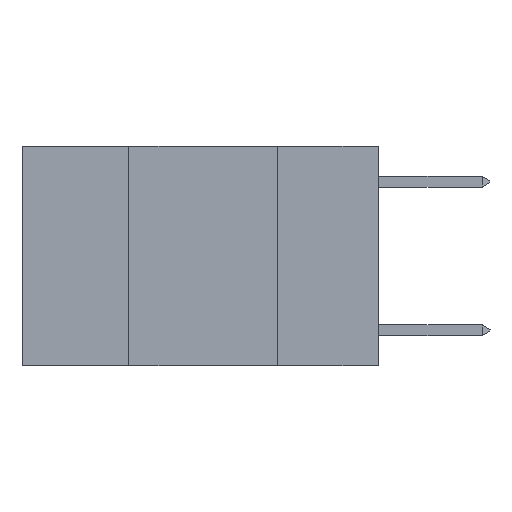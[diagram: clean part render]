
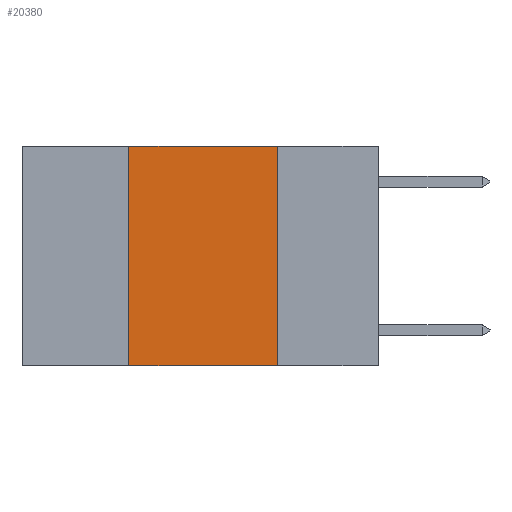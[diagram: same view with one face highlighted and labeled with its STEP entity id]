
A CAD part, left-side view. The second image highlights one B-rep face of the part: STEP entity #20380.
In plain terms, the highlighted planar face has unit normal (-1, 0, 0).
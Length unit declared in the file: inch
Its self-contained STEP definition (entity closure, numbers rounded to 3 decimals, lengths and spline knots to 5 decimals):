
#111 = DIRECTION ( 'NONE',  ( 1., 0., 0. ) ) ;
#132 = LINE ( 'NONE', #4312, #19120 ) ;
#354 = CARTESIAN_POINT ( 'NONE',  ( 0., 0.17, -0.37 ) ) ;
#672 = VERTEX_POINT ( 'NONE', #4099 ) ;
#1702 = CARTESIAN_POINT ( 'NONE',  ( 0., 0.17, 0. ) ) ;
#2691 = VECTOR ( 'NONE', #25414, 39.37008 ) ;
#3726 = DIRECTION ( 'NONE',  ( 0., 0., -1. ) ) ;
#4099 = CARTESIAN_POINT ( 'NONE',  ( 0., 0.42, 0. ) ) ;
#4312 = CARTESIAN_POINT ( 'NONE',  ( 0., 0.6, -0.37 ) ) ;
#4692 = DIRECTION ( 'NONE',  ( 0., 0., -1. ) ) ;
#7122 = LINE ( 'NONE', #19374, #2691 ) ;
#7652 = CARTESIAN_POINT ( 'NONE',  ( 0., 0.42, -0.37 ) ) ;
#8098 = ORIENTED_EDGE ( 'NONE', *, *, #11723, .T. ) ;
#8378 = DIRECTION ( 'NONE',  ( 0., -1., 0. ) ) ;
#8438 = VERTEX_POINT ( 'NONE', #354 ) ;
#8599 = EDGE_CURVE ( 'NONE', #26456, #672, #26024, .T. ) ;
#9667 = VECTOR ( 'NONE', #3726, 39.37008 ) ;
#9805 = EDGE_CURVE ( 'NONE', #672, #20671, #7122, .T. ) ;
#11723 = EDGE_CURVE ( 'NONE', #26456, #8438, #132, .T. ) ;
#13825 = DIRECTION ( 'NONE',  ( 0., 0., 1. ) ) ;
#13975 = LINE ( 'NONE', #22179, #9667 ) ;
#15125 = ORIENTED_EDGE ( 'NONE', *, *, #9805, .F. ) ;
#16006 = VECTOR ( 'NONE', #13825, 39.37008 ) ;
#17227 = AXIS2_PLACEMENT_3D ( 'NONE', #24736, #111, #4692 ) ;
#19120 = VECTOR ( 'NONE', #8378, 39.37008 ) ;
#19374 = CARTESIAN_POINT ( 'NONE',  ( 0., 0.6, 0. ) ) ;
#20332 = ORIENTED_EDGE ( 'NONE', *, *, #8599, .F. ) ;
#20380 = ADVANCED_FACE ( 'NONE', ( #20583 ), #24870, .F. ) ;
#20583 = FACE_OUTER_BOUND ( 'NONE', #25197, .T. ) ;
#20671 = VERTEX_POINT ( 'NONE', #1702 ) ;
#22179 = CARTESIAN_POINT ( 'NONE',  ( 0., 0.17, 0. ) ) ;
#23434 = EDGE_CURVE ( 'NONE', #20671, #8438, #13975, .T. ) ;
#23548 = ORIENTED_EDGE ( 'NONE', *, *, #23434, .F. ) ;
#24010 = CARTESIAN_POINT ( 'NONE',  ( 0., 0.42, 0. ) ) ;
#24736 = CARTESIAN_POINT ( 'NONE',  ( 0., 0.6, 0. ) ) ;
#24870 = PLANE ( 'NONE',  #17227 ) ;
#25197 = EDGE_LOOP ( 'NONE', ( #23548, #15125, #20332, #8098 ) ) ;
#25414 = DIRECTION ( 'NONE',  ( 0., -1., 0. ) ) ;
#26024 = LINE ( 'NONE', #24010, #16006 ) ;
#26456 = VERTEX_POINT ( 'NONE', #7652 ) ;
